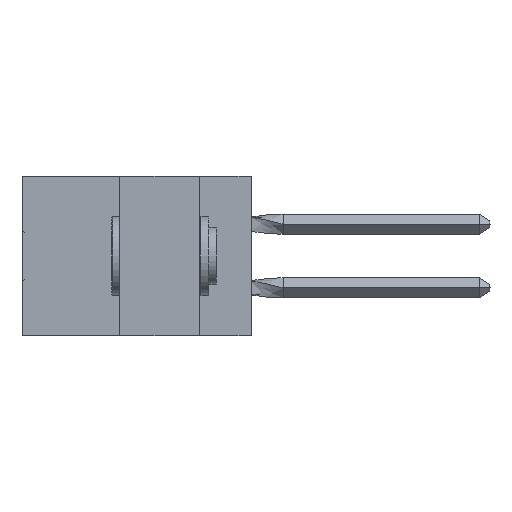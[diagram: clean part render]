
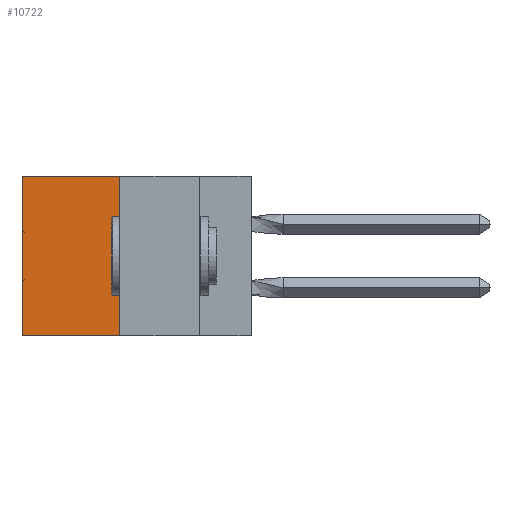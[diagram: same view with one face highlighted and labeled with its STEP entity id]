
A CAD part, left-side view. The second image highlights one B-rep face of the part: STEP entity #10722.
In plain terms, the highlighted planar face has unit normal (-1, 0, 0).
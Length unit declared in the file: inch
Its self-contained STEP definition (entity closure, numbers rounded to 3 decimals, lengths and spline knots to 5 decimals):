
#678 = CARTESIAN_POINT ( 'NONE',  ( 0.305, 0.413, -0.5 ) ) ;
#1271 = LINE ( 'NONE', #13451, #38115 ) ;
#2893 = CARTESIAN_POINT ( 'NONE',  ( 0.305, 0.413, -0.5 ) ) ;
#4235 = VERTEX_POINT ( 'NONE', #6890 ) ;
#4617 = CARTESIAN_POINT ( 'NONE',  ( 0.305, 0.72, -0.5 ) ) ;
#5825 = VECTOR ( 'NONE', #39308, 39.37008 ) ;
#6890 = CARTESIAN_POINT ( 'NONE',  ( 0.305, 0.413, 0. ) ) ;
#9547 = CARTESIAN_POINT ( 'NONE',  ( 0.305, 0.413, 0. ) ) ;
#9730 = LINE ( 'NONE', #42653, #49461 ) ;
#10722 = ADVANCED_FACE ( 'NONE', ( #12977 ), #16930, .F. ) ;
#12163 = EDGE_CURVE ( 'NONE', #4235, #39311, #16425, .T. ) ;
#12328 = ORIENTED_EDGE ( 'NONE', *, *, #12163, .T. ) ;
#12863 = VERTEX_POINT ( 'NONE', #4617 ) ;
#12977 = FACE_OUTER_BOUND ( 'NONE', #26733, .T. ) ;
#13451 = CARTESIAN_POINT ( 'NONE',  ( 0.305, 0.413, -0.5 ) ) ;
#16425 = LINE ( 'NONE', #9547, #35753 ) ;
#16930 = PLANE ( 'NONE',  #34509 ) ;
#21235 = EDGE_CURVE ( 'NONE', #28623, #12863, #27467, .T. ) ;
#21277 = ORIENTED_EDGE ( 'NONE', *, *, #36174, .T. ) ;
#24113 = ORIENTED_EDGE ( 'NONE', *, *, #38597, .F. ) ;
#24861 = DIRECTION ( 'NONE',  ( 1., 0., 0. ) ) ;
#25880 = CARTESIAN_POINT ( 'NONE',  ( 0.305, 0.72, 0. ) ) ;
#26733 = EDGE_LOOP ( 'NONE', ( #21277, #41903, #24113, #12328 ) ) ;
#27467 = LINE ( 'NONE', #678, #5825 ) ;
#28623 = VERTEX_POINT ( 'NONE', #2893 ) ;
#32138 = DIRECTION ( 'NONE',  ( 0., 0., -1. ) ) ;
#34509 = AXIS2_PLACEMENT_3D ( 'NONE', #36019, #24861, #32138 ) ;
#35753 = VECTOR ( 'NONE', #36844, 39.37008 ) ;
#36019 = CARTESIAN_POINT ( 'NONE',  ( 0.305, 0.413, -0.5 ) ) ;
#36174 = EDGE_CURVE ( 'NONE', #39311, #12863, #9730, .T. ) ;
#36844 = DIRECTION ( 'NONE',  ( 0., 1., 0. ) ) ;
#38115 = VECTOR ( 'NONE', #44276, 39.37008 ) ;
#38597 = EDGE_CURVE ( 'NONE', #4235, #28623, #1271, .T. ) ;
#38794 = DIRECTION ( 'NONE',  ( 0., 0., -1. ) ) ;
#39308 = DIRECTION ( 'NONE',  ( 0., 1., 0. ) ) ;
#39311 = VERTEX_POINT ( 'NONE', #25880 ) ;
#41903 = ORIENTED_EDGE ( 'NONE', *, *, #21235, .F. ) ;
#42653 = CARTESIAN_POINT ( 'NONE',  ( 0.305, 0.72, -0.5 ) ) ;
#44276 = DIRECTION ( 'NONE',  ( 0., 0., -1. ) ) ;
#49461 = VECTOR ( 'NONE', #38794, 39.37008 ) ;
